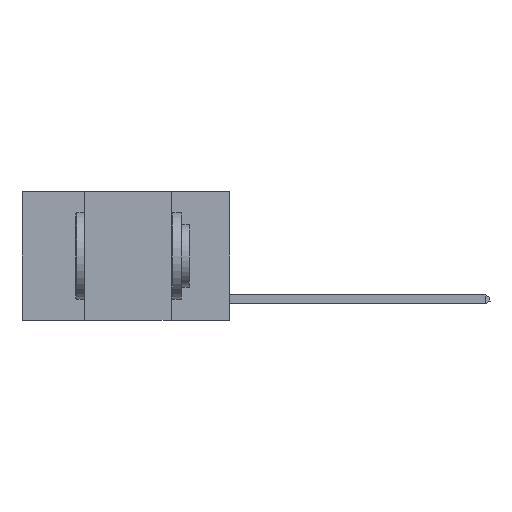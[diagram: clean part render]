
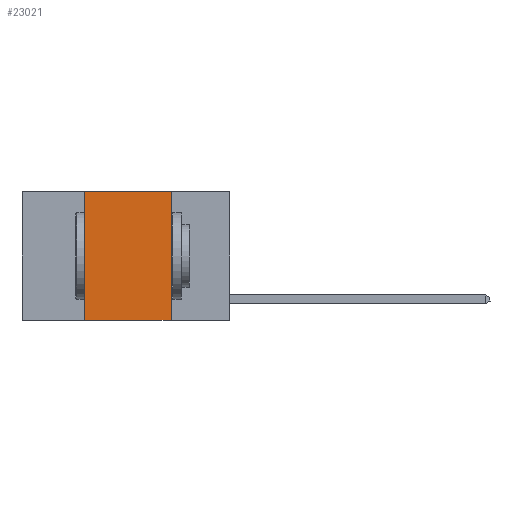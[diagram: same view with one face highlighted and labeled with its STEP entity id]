
A CAD part, left-side view. The second image highlights one B-rep face of the part: STEP entity #23021.
In plain terms, the highlighted planar face has unit normal (-1, 0, 0).
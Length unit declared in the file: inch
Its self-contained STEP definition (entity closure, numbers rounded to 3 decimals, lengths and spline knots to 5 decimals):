
#697 = VERTEX_POINT ( 'NONE', #9118 ) ;
#1389 = DIRECTION ( 'NONE',  ( 0., -1., 0. ) ) ;
#3092 = LINE ( 'NONE', #11242, #8062 ) ;
#3596 = VECTOR ( 'NONE', #9880, 39.37008 ) ;
#3817 = ORIENTED_EDGE ( 'NONE', *, *, #14492, .F. ) ;
#4669 = FACE_OUTER_BOUND ( 'NONE', #22866, .T. ) ;
#5381 = EDGE_CURVE ( 'NONE', #8204, #697, #3092, .T. ) ;
#5393 = EDGE_CURVE ( 'NONE', #18400, #16145, #17071, .T. ) ;
#5485 = ORIENTED_EDGE ( 'NONE', *, *, #5393, .F. ) ;
#5693 = EDGE_CURVE ( 'NONE', #8204, #16145, #10882, .T. ) ;
#6038 = VECTOR ( 'NONE', #1389, 39.37008 ) ;
#7667 = CARTESIAN_POINT ( 'NONE',  ( 0., 0.17, 0. ) ) ;
#8062 = VECTOR ( 'NONE', #12968, 39.37008 ) ;
#8204 = VERTEX_POINT ( 'NONE', #12139 ) ;
#8491 = PLANE ( 'NONE',  #9370 ) ;
#9118 = CARTESIAN_POINT ( 'NONE',  ( 0., 0.42, 0. ) ) ;
#9212 = VECTOR ( 'NONE', #9513, 39.37008 ) ;
#9370 = AXIS2_PLACEMENT_3D ( 'NONE', #11957, #10292, #22803 ) ;
#9513 = DIRECTION ( 'NONE',  ( 0., 0., -1. ) ) ;
#9880 = DIRECTION ( 'NONE',  ( 0., -1., 0. ) ) ;
#10292 = DIRECTION ( 'NONE',  ( 1., 0., 0. ) ) ;
#10882 = LINE ( 'NONE', #21312, #6038 ) ;
#11242 = CARTESIAN_POINT ( 'NONE',  ( 0., 0.42, 0. ) ) ;
#11957 = CARTESIAN_POINT ( 'NONE',  ( 0., 0.6, 0. ) ) ;
#12139 = CARTESIAN_POINT ( 'NONE',  ( 0., 0.42, -0.37 ) ) ;
#12902 = ORIENTED_EDGE ( 'NONE', *, *, #5381, .F. ) ;
#12968 = DIRECTION ( 'NONE',  ( 0., 0., 1. ) ) ;
#13557 = CARTESIAN_POINT ( 'NONE',  ( 0., 0.17, 0. ) ) ;
#14492 = EDGE_CURVE ( 'NONE', #697, #18400, #18098, .T. ) ;
#15214 = ORIENTED_EDGE ( 'NONE', *, *, #5693, .T. ) ;
#16145 = VERTEX_POINT ( 'NONE', #22531 ) ;
#17071 = LINE ( 'NONE', #7667, #9212 ) ;
#18098 = LINE ( 'NONE', #22388, #3596 ) ;
#18400 = VERTEX_POINT ( 'NONE', #13557 ) ;
#21312 = CARTESIAN_POINT ( 'NONE',  ( 0., 0.6, -0.37 ) ) ;
#22388 = CARTESIAN_POINT ( 'NONE',  ( 0., 0.6, 0. ) ) ;
#22531 = CARTESIAN_POINT ( 'NONE',  ( 0., 0.17, -0.37 ) ) ;
#22803 = DIRECTION ( 'NONE',  ( 0., 0., -1. ) ) ;
#22866 = EDGE_LOOP ( 'NONE', ( #5485, #3817, #12902, #15214 ) ) ;
#23021 = ADVANCED_FACE ( 'NONE', ( #4669 ), #8491, .F. ) ;
